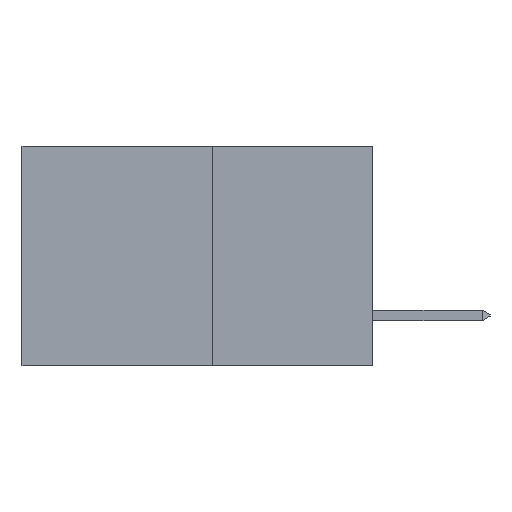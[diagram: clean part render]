
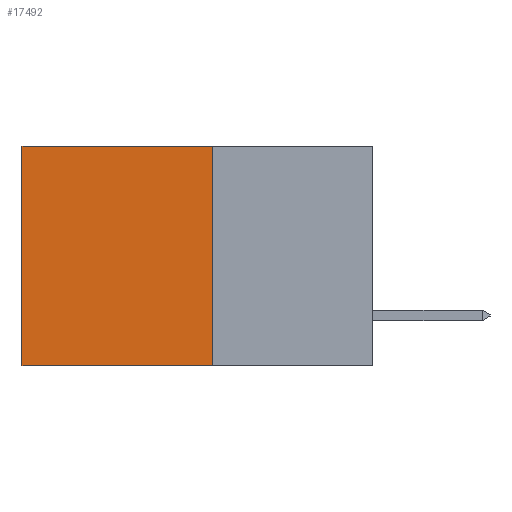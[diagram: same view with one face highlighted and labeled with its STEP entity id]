
A CAD part, left-side view. The second image highlights one B-rep face of the part: STEP entity #17492.
In plain terms, the highlighted planar face has unit normal (-1, 0, 0).
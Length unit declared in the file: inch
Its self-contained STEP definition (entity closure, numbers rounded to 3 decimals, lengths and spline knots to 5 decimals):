
#132 = ORIENTED_EDGE ( 'NONE', *, *, #1557, .F. ) ;
#673 = CARTESIAN_POINT ( 'NONE',  ( 0.277, 0.27, 0. ) ) ;
#1557 = EDGE_CURVE ( 'NONE', #17984, #12137, #15509, .T. ) ;
#2715 = VECTOR ( 'NONE', #15228, 39.37008 ) ;
#4746 = CARTESIAN_POINT ( 'NONE',  ( 0.277, 0.27, -0.37 ) ) ;
#5029 = CARTESIAN_POINT ( 'NONE',  ( 0.277, 0.27, -0.37 ) ) ;
#5258 = PLANE ( 'NONE',  #15180 ) ;
#5358 = VERTEX_POINT ( 'NONE', #10901 ) ;
#5710 = LINE ( 'NONE', #673, #14114 ) ;
#6909 = CARTESIAN_POINT ( 'NONE',  ( 0.277, 0.27, -0.37 ) ) ;
#7108 = LINE ( 'NONE', #20806, #7624 ) ;
#7624 = VECTOR ( 'NONE', #12696, 39.37008 ) ;
#7991 = VERTEX_POINT ( 'NONE', #19404 ) ;
#9648 = EDGE_LOOP ( 'NONE', ( #15242, #11687, #132, #12396 ) ) ;
#10901 = CARTESIAN_POINT ( 'NONE',  ( 0.277, 0.59, -0.37 ) ) ;
#11478 = EDGE_CURVE ( 'NONE', #7991, #5358, #12258, .T. ) ;
#11687 = ORIENTED_EDGE ( 'NONE', *, *, #20144, .F. ) ;
#12137 = VERTEX_POINT ( 'NONE', #5029 ) ;
#12258 = LINE ( 'NONE', #19748, #12784 ) ;
#12279 = DIRECTION ( 'NONE',  ( 0., 1., 0. ) ) ;
#12396 = ORIENTED_EDGE ( 'NONE', *, *, #15748, .T. ) ;
#12696 = DIRECTION ( 'NONE',  ( 0., 1., 0. ) ) ;
#12784 = VECTOR ( 'NONE', #20210, 39.37008 ) ;
#13271 = FACE_OUTER_BOUND ( 'NONE', #9648, .T. ) ;
#14114 = VECTOR ( 'NONE', #12279, 39.37008 ) ;
#15180 = AXIS2_PLACEMENT_3D ( 'NONE', #6909, #15298, #20146 ) ;
#15228 = DIRECTION ( 'NONE',  ( 0., 0., -1. ) ) ;
#15242 = ORIENTED_EDGE ( 'NONE', *, *, #11478, .T. ) ;
#15298 = DIRECTION ( 'NONE',  ( 1., 0., 0. ) ) ;
#15509 = LINE ( 'NONE', #4746, #2715 ) ;
#15748 = EDGE_CURVE ( 'NONE', #17984, #7991, #5710, .T. ) ;
#17492 = ADVANCED_FACE ( 'NONE', ( #13271 ), #5258, .F. ) ;
#17984 = VERTEX_POINT ( 'NONE', #18431 ) ;
#18431 = CARTESIAN_POINT ( 'NONE',  ( 0.277, 0.27, 0. ) ) ;
#19404 = CARTESIAN_POINT ( 'NONE',  ( 0.277, 0.59, 0. ) ) ;
#19748 = CARTESIAN_POINT ( 'NONE',  ( 0.277, 0.59, -0.37 ) ) ;
#20144 = EDGE_CURVE ( 'NONE', #12137, #5358, #7108, .T. ) ;
#20146 = DIRECTION ( 'NONE',  ( 0., 0., -1. ) ) ;
#20210 = DIRECTION ( 'NONE',  ( 0., 0., -1. ) ) ;
#20806 = CARTESIAN_POINT ( 'NONE',  ( 0.277, 0.27, -0.37 ) ) ;
